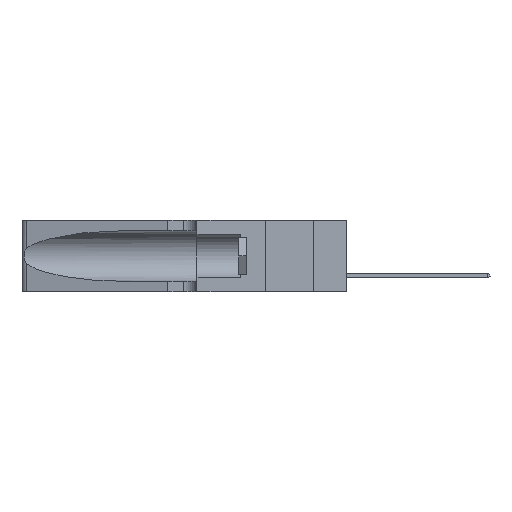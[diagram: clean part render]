
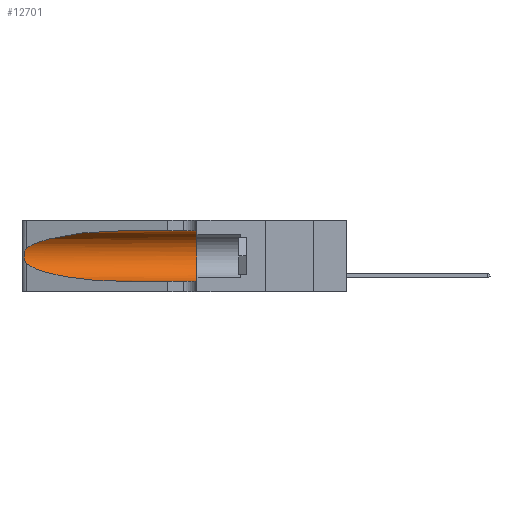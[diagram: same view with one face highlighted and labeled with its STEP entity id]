
A CAD part, left-side view. The second image highlights one B-rep face of the part: STEP entity #12701.
In plain terms, the highlighted cylindrical face has radius 3.308 mm (diameter 6.617 mm), a partial arc.
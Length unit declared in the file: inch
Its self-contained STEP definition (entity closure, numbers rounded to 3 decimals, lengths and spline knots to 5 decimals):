
#1461 = CARTESIAN_POINT ( 'NONE',  ( 0.18966, 0.96281, 0.05475 ) ) ;
#1535 = EDGE_LOOP ( 'NONE', ( #29487, #22800, #20077, #14523, #31265, #33673 ) ) ;
#2747 = CARTESIAN_POINT ( 'NONE',  ( 0.25487, 1.22718, 0.14631 ) ) ;
#4164 = CARTESIAN_POINT ( 'NONE',  ( 0.1305, 0.72297, 0.31525 ) ) ;
#4486 = CARTESIAN_POINT ( 'NONE',  ( 0.1305, 1.61858, 0.31525 ) ) ;
#4488 = CARTESIAN_POINT ( 'NONE',  ( 0.1305, 0.72297, 0.31525 ) ) ;
#4514 = LINE ( 'NONE', #18860, #5444 ) ;
#4775 =( BOUNDED_CURVE ( )  B_SPLINE_CURVE ( 3, ( #35927, #10467, #1461, #7482 ),
 .UNSPECIFIED., .F., .T. ) 
 B_SPLINE_CURVE_WITH_KNOTS ( ( 4, 4 ),
 ( 3.44316, 4.71239 ),
 .UNSPECIFIED. ) 
 CURVE ( )  GEOMETRIC_REPRESENTATION_ITEM ( )  RATIONAL_B_SPLINE_CURVE ( ( 1., 0.87, 0.87, 1. ) ) 
 REPRESENTATION_ITEM ( '' )  );
#4905 = DIRECTION ( 'NONE',  ( 0., 0., -1. ) ) ;
#5444 = VECTOR ( 'NONE', #7334, 39.37008 ) ;
#5507 = CARTESIAN_POINT ( 'NONE',  ( 0.25856, 1.23593, 0.16098 ) ) ;
#5651 = VECTOR ( 'NONE', #33840, 39.37008 ) ;
#5745 = CARTESIAN_POINT ( 'NONE',  ( 0.25639, 1.23186, 0.15144 ) ) ;
#6629 = CARTESIAN_POINT ( 'NONE',  ( 0.1305, 0.35, 0.31525 ) ) ;
#7085 = CARTESIAN_POINT ( 'NONE',  ( 0.25487, 1.22718, 0.22369 ) ) ;
#7334 = DIRECTION ( 'NONE',  ( 0., -1., 0. ) ) ;
#7421 = LINE ( 'NONE', #4486, #5651 ) ;
#7482 = CARTESIAN_POINT ( 'NONE',  ( 0.1305, 0.72297, 0.05475 ) ) ;
#7751 = VERTEX_POINT ( 'NONE', #6629 ) ;
#7773 = VERTEX_POINT ( 'NONE', #4164 ) ;
#7822 = EDGE_CURVE ( 'NONE', #19689, #26791, #4514, .T. ) ;
#9013 = CYLINDRICAL_SURFACE ( 'NONE', #12764, 0.13025 ) ;
#9514 = CARTESIAN_POINT ( 'NONE',  ( 0.1305, 0.35, 0.185 ) ) ;
#10201 = CARTESIAN_POINT ( 'NONE',  ( 0.2373, 1.15595, 0.28018 ) ) ;
#10385 = EDGE_CURVE ( 'NONE', #24717, #19689, #4775, .T. ) ;
#10467 = CARTESIAN_POINT ( 'NONE',  ( 0.2373, 1.15595, 0.08982 ) ) ;
#11125 = CARTESIAN_POINT ( 'NONE',  ( 0.26075, 1.23896, 0.178 ) ) ;
#11486 = CARTESIAN_POINT ( 'NONE',  ( 0.25555, 1.22993, 0.14849 ) ) ;
#12466 = EDGE_CURVE ( 'NONE', #14705, #24717, #35169, .T. ) ;
#12701 = ADVANCED_FACE ( 'NONE', ( #14459 ), #9013, .F. ) ;
#12764 = AXIS2_PLACEMENT_3D ( 'NONE', #36477, #30383, #4905 ) ;
#13462 = CARTESIAN_POINT ( 'NONE',  ( 0.25487, 1.22718, 0.22369 ) ) ;
#14251 = CARTESIAN_POINT ( 'NONE',  ( 0.26075, 1.23896, 0.19203 ) ) ;
#14459 = FACE_OUTER_BOUND ( 'NONE', #1535, .T. ) ;
#14523 = ORIENTED_EDGE ( 'NONE', *, *, #7822, .T. ) ;
#14705 = VERTEX_POINT ( 'NONE', #13462 ) ;
#15326 = DIRECTION ( 'NONE',  ( 0., 1., 0. ) ) ;
#17128 = CARTESIAN_POINT ( 'NONE',  ( 0.25854, 1.2359, 0.20912 ) ) ;
#17540 = EDGE_CURVE ( 'NONE', #7773, #14705, #18536, .T. ) ;
#18318 = DIRECTION ( 'NONE',  ( 0., 0., 1. ) ) ;
#18511 = CARTESIAN_POINT ( 'NONE',  ( 0.1305, 0.72297, 0.05475 ) ) ;
#18536 =( BOUNDED_CURVE ( )  B_SPLINE_CURVE ( 3, ( #4488, #30337, #10201, #7085 ),
 .UNSPECIFIED., .F., .F. ) 
 B_SPLINE_CURVE_WITH_KNOTS ( ( 4, 4 ),
 ( 1.5708, 2.84003 ),
 .UNSPECIFIED. ) 
 CURVE ( )  GEOMETRIC_REPRESENTATION_ITEM ( )  RATIONAL_B_SPLINE_CURVE ( ( 1., 0.87, 0.87, 1. ) ) 
 REPRESENTATION_ITEM ( '' )  );
#18592 = CARTESIAN_POINT ( 'NONE',  ( 0.25487, 1.22718, 0.22369 ) ) ;
#18860 = CARTESIAN_POINT ( 'NONE',  ( 0.1305, 1.61858, 0.05475 ) ) ;
#19689 = VERTEX_POINT ( 'NONE', #18511 ) ;
#20077 = ORIENTED_EDGE ( 'NONE', *, *, #10385, .T. ) ;
#21462 = CARTESIAN_POINT ( 'NONE',  ( 0.25555, 1.22994, 0.2215 ) ) ;
#22800 = ORIENTED_EDGE ( 'NONE', *, *, #12466, .T. ) ;
#22868 = CARTESIAN_POINT ( 'NONE',  ( 0.26018, 1.23835, 0.19895 ) ) ;
#24333 = CARTESIAN_POINT ( 'NONE',  ( 0.1305, 0.35, 0.05475 ) ) ;
#24717 = VERTEX_POINT ( 'NONE', #34946 ) ;
#25607 = CARTESIAN_POINT ( 'NONE',  ( 0.25639, 1.23184, 0.21858 ) ) ;
#26791 = VERTEX_POINT ( 'NONE', #24333 ) ;
#27555 = AXIS2_PLACEMENT_3D ( 'NONE', #9514, #15326, #18318 ) ;
#28254 = CARTESIAN_POINT ( 'NONE',  ( 0.26017, 1.23833, 0.17102 ) ) ;
#28482 = CARTESIAN_POINT ( 'NONE',  ( 0.25787, 1.23484, 0.2124 ) ) ;
#29487 = ORIENTED_EDGE ( 'NONE', *, *, #17540, .T. ) ;
#30337 = CARTESIAN_POINT ( 'NONE',  ( 0.18966, 0.96281, 0.31525 ) ) ;
#30383 = DIRECTION ( 'NONE',  ( 0., -1., 0. ) ) ;
#31265 = ORIENTED_EDGE ( 'NONE', *, *, #34258, .F. ) ;
#33673 = ORIENTED_EDGE ( 'NONE', *, *, #36716, .F. ) ;
#33840 = DIRECTION ( 'NONE',  ( 0., -1., 0. ) ) ;
#34106 = CARTESIAN_POINT ( 'NONE',  ( 0.25789, 1.23486, 0.15765 ) ) ;
#34258 = EDGE_CURVE ( 'NONE', #7751, #26791, #35283, .T. ) ;
#34946 = CARTESIAN_POINT ( 'NONE',  ( 0.25487, 1.22718, 0.14631 ) ) ;
#35169 = B_SPLINE_CURVE_WITH_KNOTS ( 'NONE', 3,
 ( #18592, #21462, #25607, #28482, #17128, #22868, #14251, #11125, #28254, #5507, #34106, #5745, #11486, #2747 ),
 .UNSPECIFIED., .F., .F.,
 ( 4, 2, 2, 2, 2, 2, 4 ),
 ( 0., 0.00027, 0.00053, 0.00107, 0.0016, 0.00187, 0.00214 ),
 .UNSPECIFIED. ) ;
#35283 = CIRCLE ( 'NONE', #27555, 0.13025 ) ;
#35927 = CARTESIAN_POINT ( 'NONE',  ( 0.25487, 1.22718, 0.14631 ) ) ;
#36477 = CARTESIAN_POINT ( 'NONE',  ( 0.1305, 1.61858, 0.185 ) ) ;
#36716 = EDGE_CURVE ( 'NONE', #7773, #7751, #7421, .T. ) ;
